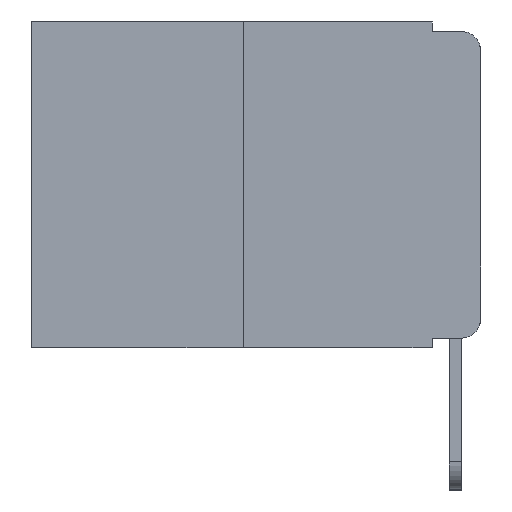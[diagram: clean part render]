
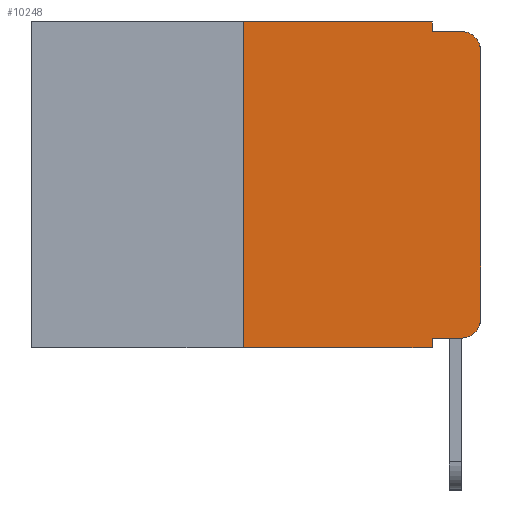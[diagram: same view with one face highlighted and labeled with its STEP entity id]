
A CAD part, left-side view. The second image highlights one B-rep face of the part: STEP entity #10248.
In plain terms, the highlighted planar face has unit normal (-1, 0, 0).
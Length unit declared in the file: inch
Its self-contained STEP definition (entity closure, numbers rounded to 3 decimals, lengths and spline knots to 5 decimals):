
#889 = CARTESIAN_POINT ( 'NONE',  ( 0., 0.473, -0.343 ) ) ;
#1200 = CARTESIAN_POINT ( 'NONE',  ( 0., 0.473, 0. ) ) ;
#1378 = VERTEX_POINT ( 'NONE', #11165 ) ;
#1520 = ORIENTED_EDGE ( 'NONE', *, *, #7757, .T. ) ;
#1532 = CARTESIAN_POINT ( 'NONE',  ( 0., 0.473, 0. ) ) ;
#1834 = VECTOR ( 'NONE', #3504, 39.37008 ) ;
#1953 = VECTOR ( 'NONE', #8347, 39.37008 ) ;
#2138 = VERTEX_POINT ( 'NONE', #7575 ) ;
#2197 = ORIENTED_EDGE ( 'NONE', *, *, #8451, .T. ) ;
#2428 = DIRECTION ( 'NONE',  ( 0., -1., 0. ) ) ;
#2475 = DIRECTION ( 'NONE',  ( 0., 0., -1. ) ) ;
#2535 = DIRECTION ( 'NONE',  ( -1., 0., 0. ) ) ;
#2568 = VERTEX_POINT ( 'NONE', #5931 ) ;
#3151 = FACE_OUTER_BOUND ( 'NONE', #6543, .T. ) ;
#3368 = CARTESIAN_POINT ( 'NONE',  ( 0., 0., -0.03 ) ) ;
#3504 = DIRECTION ( 'NONE',  ( 0., 0., -1. ) ) ;
#3582 = LINE ( 'NONE', #889, #6596 ) ;
#3886 = CARTESIAN_POINT ( 'NONE',  ( 0., 0.051, -0.333 ) ) ;
#4624 = CARTESIAN_POINT ( 'NONE',  ( 0., 0., -0.313 ) ) ;
#4645 = DIRECTION ( 'NONE',  ( 0., 0., 1. ) ) ;
#4807 = LINE ( 'NONE', #9349, #1834 ) ;
#4832 = ORIENTED_EDGE ( 'NONE', *, *, #11329, .F. ) ;
#4971 = DIRECTION ( 'NONE',  ( -1., 0., 0. ) ) ;
#5151 = VECTOR ( 'NONE', #5561, 39.37008 ) ;
#5389 = LINE ( 'NONE', #8435, #9711 ) ;
#5414 = ORIENTED_EDGE ( 'NONE', *, *, #7721, .T. ) ;
#5561 = DIRECTION ( 'NONE',  ( 0., -1., 0. ) ) ;
#5651 = CARTESIAN_POINT ( 'NONE',  ( 0., 0.051, -0.01 ) ) ;
#5666 = VERTEX_POINT ( 'NONE', #9633 ) ;
#5931 = CARTESIAN_POINT ( 'NONE',  ( 0., 0.02, -0.01 ) ) ;
#6317 = AXIS2_PLACEMENT_3D ( 'NONE', #8532, #2535, #9434 ) ;
#6334 = EDGE_CURVE ( 'NONE', #10788, #7599, #12326, .T. ) ;
#6543 = EDGE_LOOP ( 'NONE', ( #11492, #1520, #7054, #9466, #4832, #7349, #2197, #7636, #5414, #7929 ) ) ;
#6596 = VECTOR ( 'NONE', #8096, 39.37008 ) ;
#6993 = VERTEX_POINT ( 'NONE', #10883 ) ;
#7054 = ORIENTED_EDGE ( 'NONE', *, *, #7740, .F. ) ;
#7093 = CARTESIAN_POINT ( 'NONE',  ( 0., 0.051, -0.343 ) ) ;
#7349 = ORIENTED_EDGE ( 'NONE', *, *, #7724, .F. ) ;
#7575 = CARTESIAN_POINT ( 'NONE',  ( 0., 0.25, -0.343 ) ) ;
#7599 = VERTEX_POINT ( 'NONE', #3368 ) ;
#7636 = ORIENTED_EDGE ( 'NONE', *, *, #7703, .F. ) ;
#7665 = EDGE_CURVE ( 'NONE', #1378, #10788, #10822, .T. ) ;
#7670 = LINE ( 'NONE', #1200, #5151 ) ;
#7703 = EDGE_CURVE ( 'NONE', #9539, #11073, #10258, .T. ) ;
#7721 = EDGE_CURVE ( 'NONE', #9539, #1378, #12247, .T. ) ;
#7724 = EDGE_CURVE ( 'NONE', #2138, #9151, #5389, .T. ) ;
#7740 = EDGE_CURVE ( 'NONE', #6993, #2568, #11999, .T. ) ;
#7743 = EDGE_CURVE ( 'NONE', #5666, #6993, #4807, .T. ) ;
#7757 = EDGE_CURVE ( 'NONE', #7599, #2568, #11731, .T. ) ;
#7929 = ORIENTED_EDGE ( 'NONE', *, *, #7665, .T. ) ;
#8096 = DIRECTION ( 'NONE',  ( 0., -1., 0. ) ) ;
#8347 = DIRECTION ( 'NONE',  ( 0., 0., 1. ) ) ;
#8435 = CARTESIAN_POINT ( 'NONE',  ( 0., 0.25, 0. ) ) ;
#8451 = EDGE_CURVE ( 'NONE', #2138, #11073, #3582, .T. ) ;
#8532 = CARTESIAN_POINT ( 'NONE',  ( 0., 0.02, -0.03 ) ) ;
#9151 = VERTEX_POINT ( 'NONE', #10191 ) ;
#9349 = CARTESIAN_POINT ( 'NONE',  ( 0., 0.051, 0. ) ) ;
#9434 = DIRECTION ( 'NONE',  ( 0., 0., -1. ) ) ;
#9449 = VECTOR ( 'NONE', #2428, 39.37008 ) ;
#9466 = ORIENTED_EDGE ( 'NONE', *, *, #7743, .F. ) ;
#9539 = VERTEX_POINT ( 'NONE', #3886 ) ;
#9633 = CARTESIAN_POINT ( 'NONE',  ( 0., 0.051, 0. ) ) ;
#9711 = VECTOR ( 'NONE', #4645, 39.37008 ) ;
#9714 = AXIS2_PLACEMENT_3D ( 'NONE', #1532, #10376, #2475 ) ;
#10191 = CARTESIAN_POINT ( 'NONE',  ( 0., 0.25, 0. ) ) ;
#10248 = ADVANCED_FACE ( 'NONE', ( #3151 ), #12048, .F. ) ;
#10258 = LINE ( 'NONE', #12315, #10538 ) ;
#10376 = DIRECTION ( 'NONE',  ( 1., 0., 0. ) ) ;
#10538 = VECTOR ( 'NONE', #11996, 39.37008 ) ;
#10788 = VERTEX_POINT ( 'NONE', #4624 ) ;
#10804 = CARTESIAN_POINT ( 'NONE',  ( 0., 0., 0. ) ) ;
#10822 = CIRCLE ( 'NONE', #12078, 0.02 ) ;
#10883 = CARTESIAN_POINT ( 'NONE',  ( 0., 0.051, -0.01 ) ) ;
#11073 = VERTEX_POINT ( 'NONE', #7093 ) ;
#11165 = CARTESIAN_POINT ( 'NONE',  ( 0., 0.02, -0.333 ) ) ;
#11329 = EDGE_CURVE ( 'NONE', #9151, #5666, #7670, .T. ) ;
#11492 = ORIENTED_EDGE ( 'NONE', *, *, #6334, .T. ) ;
#11604 = CARTESIAN_POINT ( 'NONE',  ( 0., 0.02, -0.313 ) ) ;
#11731 = CIRCLE ( 'NONE', #6317, 0.02 ) ;
#11873 = DIRECTION ( 'NONE',  ( 0., -1., 0. ) ) ;
#11996 = DIRECTION ( 'NONE',  ( 0., 0., -1. ) ) ;
#11999 = LINE ( 'NONE', #5651, #9449 ) ;
#12048 = PLANE ( 'NONE',  #9714 ) ;
#12078 = AXIS2_PLACEMENT_3D ( 'NONE', #11604, #4971, #12309 ) ;
#12247 = LINE ( 'NONE', #12444, #12493 ) ;
#12309 = DIRECTION ( 'NONE',  ( 0., 0., -1. ) ) ;
#12315 = CARTESIAN_POINT ( 'NONE',  ( 0., 0.051, 0. ) ) ;
#12326 = LINE ( 'NONE', #10804, #1953 ) ;
#12444 = CARTESIAN_POINT ( 'NONE',  ( 0., 0.051, -0.333 ) ) ;
#12493 = VECTOR ( 'NONE', #11873, 39.37008 ) ;
